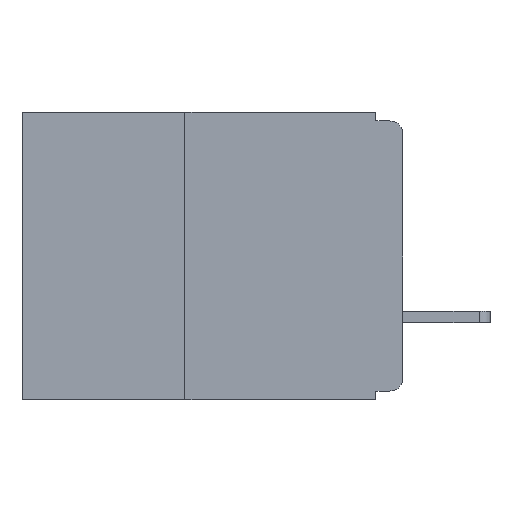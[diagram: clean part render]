
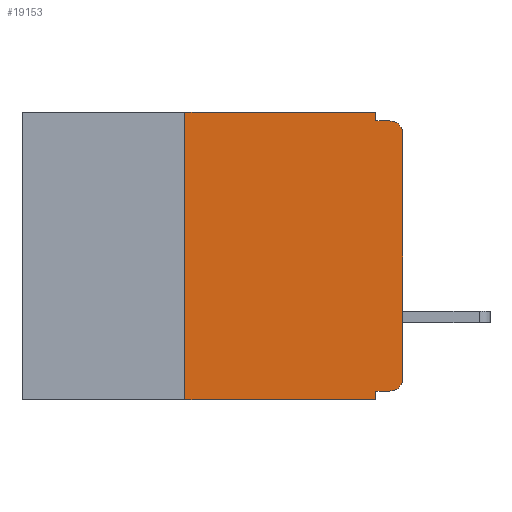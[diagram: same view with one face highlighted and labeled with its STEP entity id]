
A CAD part, left-side view. The second image highlights one B-rep face of the part: STEP entity #19153.
In plain terms, the highlighted planar face has unit normal (-1, 0, 0).
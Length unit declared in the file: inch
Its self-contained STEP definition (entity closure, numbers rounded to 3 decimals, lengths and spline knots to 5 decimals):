
#269 = ORIENTED_EDGE ( 'NONE', *, *, #16422, .F. ) ;
#635 = CARTESIAN_POINT ( 'NONE',  ( 0., 0.031, 0. ) ) ;
#1070 = CARTESIAN_POINT ( 'NONE',  ( 0., 0.437, -0.33 ) ) ;
#1204 = CARTESIAN_POINT ( 'NONE',  ( 0., 0.015, -0.32 ) ) ;
#1259 = VERTEX_POINT ( 'NONE', #6136 ) ;
#1602 = CARTESIAN_POINT ( 'NONE',  ( 0., 0.437, 0. ) ) ;
#1832 = AXIS2_PLACEMENT_3D ( 'NONE', #1602, #5059, #17182 ) ;
#1897 = ORIENTED_EDGE ( 'NONE', *, *, #2117, .F. ) ;
#2095 = VERTEX_POINT ( 'NONE', #13825 ) ;
#2117 = EDGE_CURVE ( 'NONE', #3047, #2880, #20944, .T. ) ;
#2169 = DIRECTION ( 'NONE',  ( 0., -1., 0. ) ) ;
#2394 = DIRECTION ( 'NONE',  ( 0., 0., -1. ) ) ;
#2419 = DIRECTION ( 'NONE',  ( -1., 0., 0. ) ) ;
#2427 = VERTEX_POINT ( 'NONE', #21564 ) ;
#2540 = CARTESIAN_POINT ( 'NONE',  ( 0., 0.015, -0.025 ) ) ;
#2815 = DIRECTION ( 'NONE',  ( 0., -1., 0. ) ) ;
#2880 = VERTEX_POINT ( 'NONE', #4891 ) ;
#2971 = VERTEX_POINT ( 'NONE', #1204 ) ;
#2989 = CARTESIAN_POINT ( 'NONE',  ( 0., 0., -0.025 ) ) ;
#3047 = VERTEX_POINT ( 'NONE', #20898 ) ;
#3330 = PLANE ( 'NONE',  #1832 ) ;
#3792 = ORIENTED_EDGE ( 'NONE', *, *, #10175, .T. ) ;
#4343 = LINE ( 'NONE', #10870, #13032 ) ;
#4891 = CARTESIAN_POINT ( 'NONE',  ( 0., 0.031, -0.33 ) ) ;
#5059 = DIRECTION ( 'NONE',  ( 1., 0., 0. ) ) ;
#5826 = AXIS2_PLACEMENT_3D ( 'NONE', #2540, #2419, #2394 ) ;
#5947 = ORIENTED_EDGE ( 'NONE', *, *, #8884, .T. ) ;
#6136 = CARTESIAN_POINT ( 'NONE',  ( 0., 0.031, 0. ) ) ;
#6207 = EDGE_CURVE ( 'NONE', #21983, #2427, #16585, .T. ) ;
#6345 = LINE ( 'NONE', #17676, #10444 ) ;
#7273 = CARTESIAN_POINT ( 'NONE',  ( 0., 0.031, -0.01 ) ) ;
#7284 = VERTEX_POINT ( 'NONE', #9983 ) ;
#7331 = VECTOR ( 'NONE', #8809, 39.37008 ) ;
#8809 = DIRECTION ( 'NONE',  ( 0., 1., 0. ) ) ;
#8884 = EDGE_CURVE ( 'NONE', #7284, #2880, #9090, .T. ) ;
#9037 = VECTOR ( 'NONE', #11885, 39.37008 ) ;
#9090 = LINE ( 'NONE', #1070, #17777 ) ;
#9605 = LINE ( 'NONE', #18719, #9037 ) ;
#9983 = CARTESIAN_POINT ( 'NONE',  ( 0., 0.25, -0.33 ) ) ;
#10018 = ORIENTED_EDGE ( 'NONE', *, *, #16888, .F. ) ;
#10175 = EDGE_CURVE ( 'NONE', #16908, #21983, #11670, .T. ) ;
#10253 = CARTESIAN_POINT ( 'NONE',  ( 0., 0.015, -0.305 ) ) ;
#10354 = EDGE_CURVE ( 'NONE', #2971, #16908, #20515, .T. ) ;
#10444 = VECTOR ( 'NONE', #2169, 39.37008 ) ;
#10677 = CARTESIAN_POINT ( 'NONE',  ( 0., 0., -0.32 ) ) ;
#10870 = CARTESIAN_POINT ( 'NONE',  ( 0., 0.25, -0.33 ) ) ;
#11048 = FACE_OUTER_BOUND ( 'NONE', #19464, .T. ) ;
#11130 = ORIENTED_EDGE ( 'NONE', *, *, #21703, .F. ) ;
#11670 = LINE ( 'NONE', #19976, #18664 ) ;
#11672 = ORIENTED_EDGE ( 'NONE', *, *, #10354, .T. ) ;
#11856 = VECTOR ( 'NONE', #14452, 39.37008 ) ;
#11885 = DIRECTION ( 'NONE',  ( 0., -1., 0. ) ) ;
#12025 = DIRECTION ( 'NONE',  ( 0., 0., -1. ) ) ;
#12617 = DIRECTION ( 'NONE',  ( 0., 0., 1. ) ) ;
#12725 = EDGE_CURVE ( 'NONE', #2095, #1259, #6345, .T. ) ;
#13032 = VECTOR ( 'NONE', #12617, 39.37008 ) ;
#13574 = ORIENTED_EDGE ( 'NONE', *, *, #20400, .F. ) ;
#13624 = CARTESIAN_POINT ( 'NONE',  ( 0., 0.031, -0.33 ) ) ;
#13825 = CARTESIAN_POINT ( 'NONE',  ( 0., 0.25, 0. ) ) ;
#14452 = DIRECTION ( 'NONE',  ( 0., 0., -1. ) ) ;
#14517 = DIRECTION ( 'NONE',  ( 0., 0., -1. ) ) ;
#14670 = VECTOR ( 'NONE', #14517, 39.37008 ) ;
#16422 = EDGE_CURVE ( 'NONE', #1259, #18144, #19228, .T. ) ;
#16585 = CIRCLE ( 'NONE', #5826, 0.015 ) ;
#16600 = LINE ( 'NONE', #10677, #7331 ) ;
#16888 = EDGE_CURVE ( 'NONE', #7284, #2095, #4343, .T. ) ;
#16908 = VERTEX_POINT ( 'NONE', #17803 ) ;
#17182 = DIRECTION ( 'NONE',  ( 0., 0., -1. ) ) ;
#17676 = CARTESIAN_POINT ( 'NONE',  ( 0., 0.437, 0. ) ) ;
#17777 = VECTOR ( 'NONE', #2815, 39.37008 ) ;
#17803 = CARTESIAN_POINT ( 'NONE',  ( 0., 0., -0.305 ) ) ;
#18144 = VERTEX_POINT ( 'NONE', #7273 ) ;
#18334 = DIRECTION ( 'NONE',  ( 0., 0., 1. ) ) ;
#18664 = VECTOR ( 'NONE', #18334, 39.37008 ) ;
#18666 = ORIENTED_EDGE ( 'NONE', *, *, #12725, .F. ) ;
#18719 = CARTESIAN_POINT ( 'NONE',  ( 0., 0., -0.01 ) ) ;
#19153 = ADVANCED_FACE ( 'NONE', ( #11048 ), #3330, .F. ) ;
#19228 = LINE ( 'NONE', #635, #14670 ) ;
#19464 = EDGE_LOOP ( 'NONE', ( #3792, #22063, #13574, #269, #18666, #10018, #5947, #1897, #11130, #11672 ) ) ;
#19976 = CARTESIAN_POINT ( 'NONE',  ( 0., 0., 0. ) ) ;
#20400 = EDGE_CURVE ( 'NONE', #18144, #2427, #9605, .T. ) ;
#20515 = CIRCLE ( 'NONE', #21709, 0.015 ) ;
#20898 = CARTESIAN_POINT ( 'NONE',  ( 0., 0.031, -0.32 ) ) ;
#20944 = LINE ( 'NONE', #13624, #11856 ) ;
#21564 = CARTESIAN_POINT ( 'NONE',  ( 0., 0.015, -0.01 ) ) ;
#21703 = EDGE_CURVE ( 'NONE', #2971, #3047, #16600, .T. ) ;
#21709 = AXIS2_PLACEMENT_3D ( 'NONE', #10253, #22208, #12025 ) ;
#21983 = VERTEX_POINT ( 'NONE', #2989 ) ;
#22063 = ORIENTED_EDGE ( 'NONE', *, *, #6207, .T. ) ;
#22208 = DIRECTION ( 'NONE',  ( -1., 0., 0. ) ) ;
